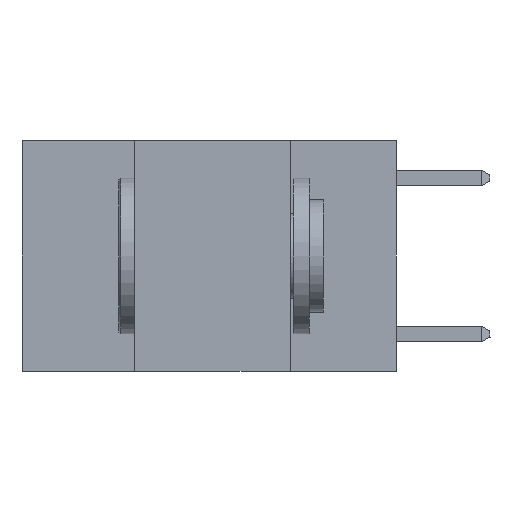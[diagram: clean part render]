
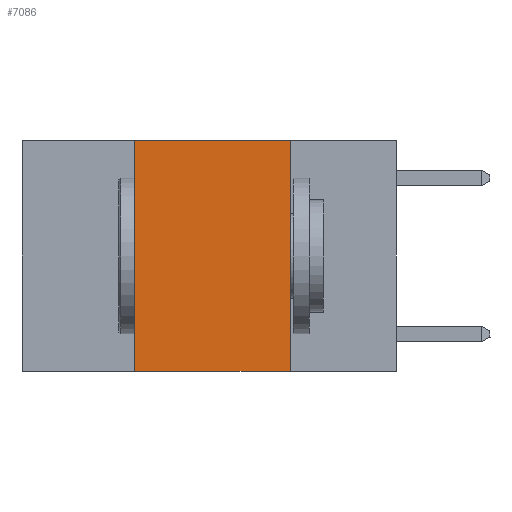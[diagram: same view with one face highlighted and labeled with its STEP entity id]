
A CAD part, left-side view. The second image highlights one B-rep face of the part: STEP entity #7086.
In plain terms, the highlighted planar face has unit normal (-1, 0, 0).
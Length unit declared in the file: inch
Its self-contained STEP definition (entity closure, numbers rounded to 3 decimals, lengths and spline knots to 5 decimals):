
#322 = CARTESIAN_POINT ( 'NONE',  ( 0., 0.6, -0.37 ) ) ;
#410 = EDGE_CURVE ( 'NONE', #7355, #6271, #8661, .T. ) ;
#513 = DIRECTION ( 'NONE',  ( 0., -1., 0. ) ) ;
#571 = VECTOR ( 'NONE', #4723, 39.37008 ) ;
#639 = CARTESIAN_POINT ( 'NONE',  ( 0., 0.6, 0. ) ) ;
#744 = AXIS2_PLACEMENT_3D ( 'NONE', #2665, #7012, #4259 ) ;
#1333 = CARTESIAN_POINT ( 'NONE',  ( 0., 0.42, 0. ) ) ;
#1475 = CARTESIAN_POINT ( 'NONE',  ( 0., 0.42, -0.37 ) ) ;
#2172 = CARTESIAN_POINT ( 'NONE',  ( 0., 0.42, 0. ) ) ;
#2345 = VERTEX_POINT ( 'NONE', #11220 ) ;
#2665 = CARTESIAN_POINT ( 'NONE',  ( 0., 0.6, 0. ) ) ;
#3451 = VERTEX_POINT ( 'NONE', #1475 ) ;
#3731 = LINE ( 'NONE', #322, #571 ) ;
#3785 = EDGE_LOOP ( 'NONE', ( #8744, #8301, #9155, #8492 ) ) ;
#4259 = DIRECTION ( 'NONE',  ( 0., 0., -1. ) ) ;
#4723 = DIRECTION ( 'NONE',  ( 0., -1., 0. ) ) ;
#5783 = DIRECTION ( 'NONE',  ( 0., 0., 1. ) ) ;
#5896 = LINE ( 'NONE', #1333, #9902 ) ;
#6225 = LINE ( 'NONE', #9576, #8987 ) ;
#6271 = VERTEX_POINT ( 'NONE', #8631 ) ;
#7012 = DIRECTION ( 'NONE',  ( 1., 0., 0. ) ) ;
#7017 = EDGE_CURVE ( 'NONE', #3451, #7355, #5896, .T. ) ;
#7086 = ADVANCED_FACE ( 'NONE', ( #10592 ), #9644, .F. ) ;
#7355 = VERTEX_POINT ( 'NONE', #2172 ) ;
#8301 = ORIENTED_EDGE ( 'NONE', *, *, #410, .F. ) ;
#8492 = ORIENTED_EDGE ( 'NONE', *, *, #9027, .T. ) ;
#8631 = CARTESIAN_POINT ( 'NONE',  ( 0., 0.17, 0. ) ) ;
#8661 = LINE ( 'NONE', #639, #8851 ) ;
#8684 = EDGE_CURVE ( 'NONE', #6271, #2345, #6225, .T. ) ;
#8744 = ORIENTED_EDGE ( 'NONE', *, *, #8684, .F. ) ;
#8766 = DIRECTION ( 'NONE',  ( 0., 0., -1. ) ) ;
#8851 = VECTOR ( 'NONE', #513, 39.37008 ) ;
#8987 = VECTOR ( 'NONE', #8766, 39.37008 ) ;
#9027 = EDGE_CURVE ( 'NONE', #3451, #2345, #3731, .T. ) ;
#9155 = ORIENTED_EDGE ( 'NONE', *, *, #7017, .F. ) ;
#9576 = CARTESIAN_POINT ( 'NONE',  ( 0., 0.17, 0. ) ) ;
#9644 = PLANE ( 'NONE',  #744 ) ;
#9902 = VECTOR ( 'NONE', #5783, 39.37008 ) ;
#10592 = FACE_OUTER_BOUND ( 'NONE', #3785, .T. ) ;
#11220 = CARTESIAN_POINT ( 'NONE',  ( 0., 0.17, -0.37 ) ) ;
